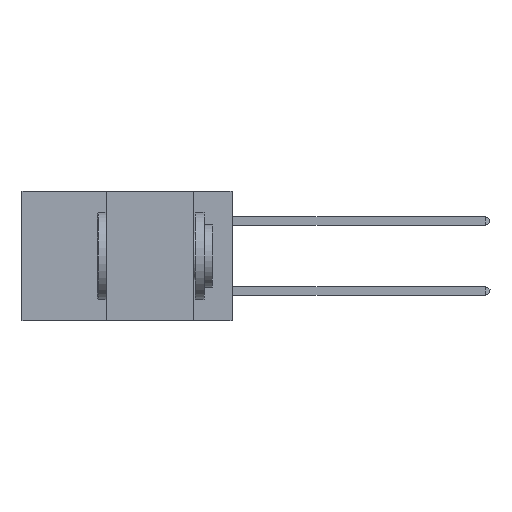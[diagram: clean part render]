
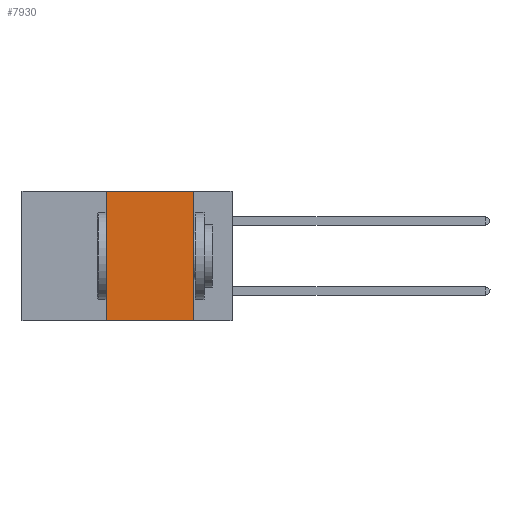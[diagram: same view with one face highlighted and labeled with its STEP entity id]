
A CAD part, left-side view. The second image highlights one B-rep face of the part: STEP entity #7930.
In plain terms, the highlighted planar face has unit normal (-1, 0, 0).
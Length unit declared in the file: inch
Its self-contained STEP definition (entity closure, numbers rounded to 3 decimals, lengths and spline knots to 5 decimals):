
#162 = CARTESIAN_POINT ( 'NONE',  ( 0., 0.6, -0.37 ) ) ;
#403 = DIRECTION ( 'NONE',  ( 0., 0., -1. ) ) ;
#599 = DIRECTION ( 'NONE',  ( 0., 0., -1. ) ) ;
#1396 = CARTESIAN_POINT ( 'NONE',  ( 0., 0.36, -0.37 ) ) ;
#2185 = ORIENTED_EDGE ( 'NONE', *, *, #14851, .T. ) ;
#2337 = AXIS2_PLACEMENT_3D ( 'NONE', #3982, #7710, #403 ) ;
#2602 = VERTEX_POINT ( 'NONE', #14273 ) ;
#2634 = EDGE_CURVE ( 'NONE', #12406, #5053, #5554, .T. ) ;
#3591 = LINE ( 'NONE', #12108, #6362 ) ;
#3646 = VECTOR ( 'NONE', #4078, 39.37008 ) ;
#3769 = EDGE_LOOP ( 'NONE', ( #10482, #4821, #10648, #2185 ) ) ;
#3982 = CARTESIAN_POINT ( 'NONE',  ( 0., 0.6, 0. ) ) ;
#4078 = DIRECTION ( 'NONE',  ( 0., -1., 0. ) ) ;
#4674 = DIRECTION ( 'NONE',  ( 0., 0., 1. ) ) ;
#4686 = CARTESIAN_POINT ( 'NONE',  ( 0., 0.11, 0. ) ) ;
#4821 = ORIENTED_EDGE ( 'NONE', *, *, #5799, .F. ) ;
#4839 = LINE ( 'NONE', #11637, #3646 ) ;
#5053 = VERTEX_POINT ( 'NONE', #14889 ) ;
#5554 = LINE ( 'NONE', #12983, #8543 ) ;
#5799 = EDGE_CURVE ( 'NONE', #2602, #12406, #4839, .T. ) ;
#6362 = VECTOR ( 'NONE', #4674, 39.37008 ) ;
#7710 = DIRECTION ( 'NONE',  ( 1., 0., 0. ) ) ;
#7930 = ADVANCED_FACE ( 'NONE', ( #12389 ), #11545, .F. ) ;
#8543 = VECTOR ( 'NONE', #599, 39.37008 ) ;
#8963 = DIRECTION ( 'NONE',  ( 0., -1., 0. ) ) ;
#9239 = VECTOR ( 'NONE', #8963, 39.37008 ) ;
#10482 = ORIENTED_EDGE ( 'NONE', *, *, #2634, .F. ) ;
#10648 = ORIENTED_EDGE ( 'NONE', *, *, #12835, .F. ) ;
#10992 = VERTEX_POINT ( 'NONE', #1396 ) ;
#11545 = PLANE ( 'NONE',  #2337 ) ;
#11637 = CARTESIAN_POINT ( 'NONE',  ( 0., 0.6, 0. ) ) ;
#12108 = CARTESIAN_POINT ( 'NONE',  ( 0., 0.36, 0. ) ) ;
#12389 = FACE_OUTER_BOUND ( 'NONE', #3769, .T. ) ;
#12406 = VERTEX_POINT ( 'NONE', #4686 ) ;
#12835 = EDGE_CURVE ( 'NONE', #10992, #2602, #3591, .T. ) ;
#12983 = CARTESIAN_POINT ( 'NONE',  ( 0., 0.11, 0. ) ) ;
#14273 = CARTESIAN_POINT ( 'NONE',  ( 0., 0.36, 0. ) ) ;
#14851 = EDGE_CURVE ( 'NONE', #10992, #5053, #16063, .T. ) ;
#14889 = CARTESIAN_POINT ( 'NONE',  ( 0., 0.11, -0.37 ) ) ;
#16063 = LINE ( 'NONE', #162, #9239 ) ;
